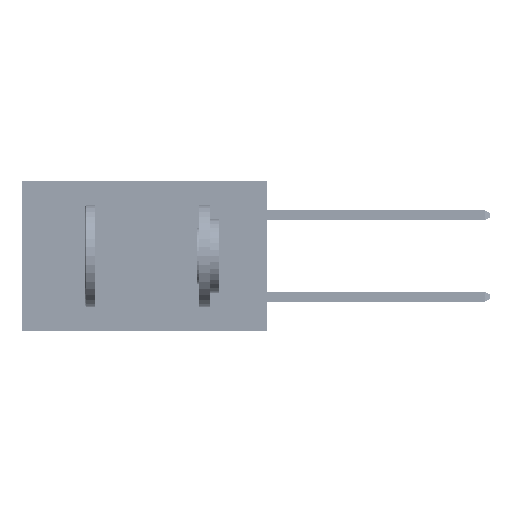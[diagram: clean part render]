
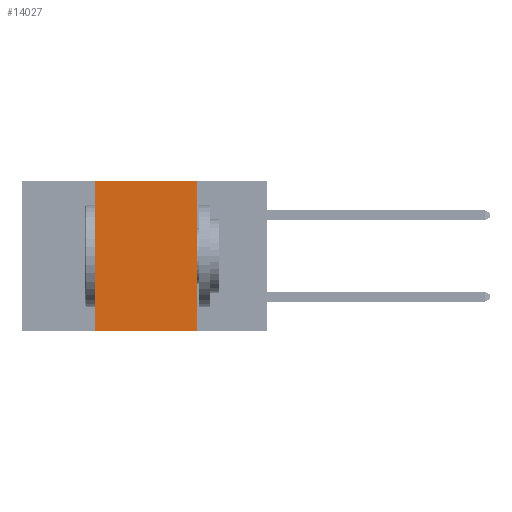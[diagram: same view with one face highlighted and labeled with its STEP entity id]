
A CAD part, left-side view. The second image highlights one B-rep face of the part: STEP entity #14027.
In plain terms, the highlighted planar face has unit normal (-1, 0, 0).
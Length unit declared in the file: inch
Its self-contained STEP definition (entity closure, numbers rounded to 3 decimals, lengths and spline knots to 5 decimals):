
#2406 = EDGE_CURVE ( 'NONE', #42539, #21760, #38494, .T. ) ;
#3720 = CARTESIAN_POINT ( 'NONE',  ( 0., 0.17, 0. ) ) ;
#3959 = VERTEX_POINT ( 'NONE', #25974 ) ;
#5026 = CARTESIAN_POINT ( 'NONE',  ( 0., 0.6, 0. ) ) ;
#6697 = ORIENTED_EDGE ( 'NONE', *, *, #32349, .F. ) ;
#7518 = DIRECTION ( 'NONE',  ( 0., 0., 1. ) ) ;
#9442 = VECTOR ( 'NONE', #7518, 39.37008 ) ;
#13649 = CARTESIAN_POINT ( 'NONE',  ( 0., 0.17, 0. ) ) ;
#14027 = ADVANCED_FACE ( 'NONE', ( #23670 ), #18068, .F. ) ;
#14357 = LINE ( 'NONE', #27347, #9442 ) ;
#18068 = PLANE ( 'NONE',  #20335 ) ;
#18165 = ORIENTED_EDGE ( 'NONE', *, *, #30323, .F. ) ;
#18202 = EDGE_LOOP ( 'NONE', ( #6697, #34461, #18165, #28978 ) ) ;
#20335 = AXIS2_PLACEMENT_3D ( 'NONE', #45820, #22008, #33812 ) ;
#21760 = VERTEX_POINT ( 'NONE', #13649 ) ;
#22008 = DIRECTION ( 'NONE',  ( 1., 0., 0. ) ) ;
#22079 = VECTOR ( 'NONE', #43506, 39.37008 ) ;
#22249 = VECTOR ( 'NONE', #36895, 39.37008 ) ;
#23670 = FACE_OUTER_BOUND ( 'NONE', #18202, .T. ) ;
#25974 = CARTESIAN_POINT ( 'NONE',  ( 0., 0.17, -0.37 ) ) ;
#27347 = CARTESIAN_POINT ( 'NONE',  ( 0., 0.42, 0. ) ) ;
#28978 = ORIENTED_EDGE ( 'NONE', *, *, #50470, .T. ) ;
#30323 = EDGE_CURVE ( 'NONE', #44799, #42539, #14357, .T. ) ;
#32349 = EDGE_CURVE ( 'NONE', #21760, #3959, #40469, .T. ) ;
#33067 = CARTESIAN_POINT ( 'NONE',  ( 0., 0.42, 0. ) ) ;
#33812 = DIRECTION ( 'NONE',  ( 0., 0., -1. ) ) ;
#34461 = ORIENTED_EDGE ( 'NONE', *, *, #2406, .F. ) ;
#35256 = CARTESIAN_POINT ( 'NONE',  ( 0., 0.42, -0.37 ) ) ;
#36895 = DIRECTION ( 'NONE',  ( 0., -1., 0. ) ) ;
#38494 = LINE ( 'NONE', #5026, #45247 ) ;
#40202 = CARTESIAN_POINT ( 'NONE',  ( 0., 0.6, -0.37 ) ) ;
#40469 = LINE ( 'NONE', #3720, #22079 ) ;
#41535 = DIRECTION ( 'NONE',  ( 0., -1., 0. ) ) ;
#42539 = VERTEX_POINT ( 'NONE', #33067 ) ;
#43506 = DIRECTION ( 'NONE',  ( 0., 0., -1. ) ) ;
#44799 = VERTEX_POINT ( 'NONE', #35256 ) ;
#45247 = VECTOR ( 'NONE', #41535, 39.37008 ) ;
#45820 = CARTESIAN_POINT ( 'NONE',  ( 0., 0.6, 0. ) ) ;
#46754 = LINE ( 'NONE', #40202, #22249 ) ;
#50470 = EDGE_CURVE ( 'NONE', #44799, #3959, #46754, .T. ) ;
